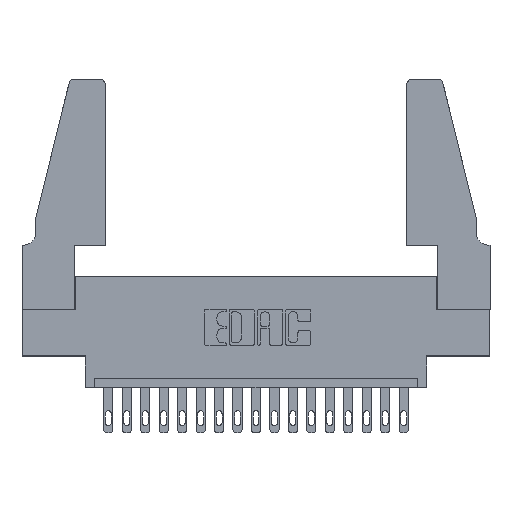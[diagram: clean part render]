
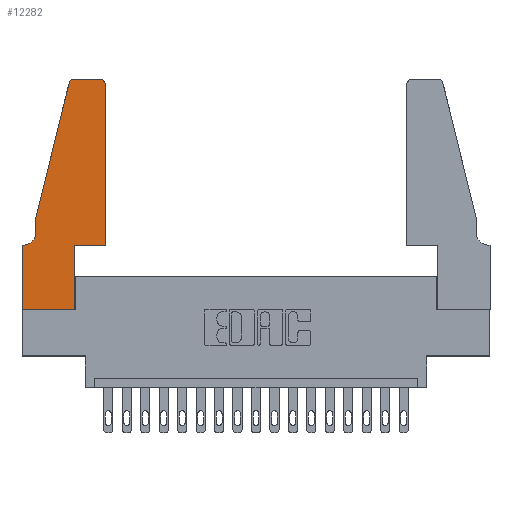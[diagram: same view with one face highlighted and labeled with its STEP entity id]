
A CAD part, top view. The second image highlights one B-rep face of the part: STEP entity #12282.
In plain terms, the highlighted planar face has unit normal (0, 0, 1).
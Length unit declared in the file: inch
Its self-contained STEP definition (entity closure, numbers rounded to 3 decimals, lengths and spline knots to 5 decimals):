
#371 = VECTOR ( 'NONE', #3608, 39.37008 ) ;
#410 = VERTEX_POINT ( 'NONE', #6914 ) ;
#624 = ORIENTED_EDGE ( 'NONE', *, *, #14106, .T. ) ;
#739 = CARTESIAN_POINT ( 'NONE',  ( 0.2865, 0.35, 0.37 ) ) ;
#763 = VERTEX_POINT ( 'NONE', #1610 ) ;
#771 = CARTESIAN_POINT ( 'NONE',  ( 0.4505, 0.35, 0.37 ) ) ;
#846 = LINE ( 'NONE', #1832, #3275 ) ;
#1291 = CARTESIAN_POINT ( 'NONE',  ( 0.0755, 0.5, 0.37 ) ) ;
#1357 = CARTESIAN_POINT ( 'NONE',  ( 0., 0., 0.37 ) ) ;
#1410 = CARTESIAN_POINT ( 'NONE',  ( 0.2865, 0.35, 0.37 ) ) ;
#1493 = CARTESIAN_POINT ( 'NONE',  ( 0.4505, 0.35, 0.37 ) ) ;
#1610 = CARTESIAN_POINT ( 'NONE',  ( 0.25487, 1.22718, 0.37 ) ) ;
#1832 = CARTESIAN_POINT ( 'NONE',  ( 0.2605, 1.25, 0.37 ) ) ;
#1954 = EDGE_CURVE ( 'NONE', #10099, #12650, #4703, .T. ) ;
#2339 = DIRECTION ( 'NONE',  ( 1., 0., 0. ) ) ;
#2361 = VECTOR ( 'NONE', #6829, 39.37008 ) ;
#2858 = ORIENTED_EDGE ( 'NONE', *, *, #18289, .T. ) ;
#3275 = VECTOR ( 'NONE', #7366, 39.37008 ) ;
#3564 = ORIENTED_EDGE ( 'NONE', *, *, #7827, .T. ) ;
#3608 = DIRECTION ( 'NONE',  ( 0., 1., 0. ) ) ;
#3781 = CARTESIAN_POINT ( 'NONE',  ( 0., 0., 0.37 ) ) ;
#3797 = AXIS2_PLACEMENT_3D ( 'NONE', #14997, #4817, #7934 ) ;
#4042 = LINE ( 'NONE', #10517, #10256 ) ;
#4330 = EDGE_CURVE ( 'NONE', #6242, #4493, #17198, .T. ) ;
#4493 = VERTEX_POINT ( 'NONE', #7048 ) ;
#4703 = CIRCLE ( 'NONE', #17591, 0.07 ) ;
#4817 = DIRECTION ( 'NONE',  ( 0., 0., 1. ) ) ;
#4842 = DIRECTION ( 'NONE',  ( 1., 0., 0. ) ) ;
#5022 = VECTOR ( 'NONE', #16848, 39.37008 ) ;
#5751 = LINE ( 'NONE', #18090, #9321 ) ;
#6242 = VERTEX_POINT ( 'NONE', #771 ) ;
#6408 = DIRECTION ( 'NONE',  ( 0., 0., 1. ) ) ;
#6492 = PLANE ( 'NONE',  #8115 ) ;
#6562 = VECTOR ( 'NONE', #10854, 39.37008 ) ;
#6829 = DIRECTION ( 'NONE',  ( -0.239, -0.971, 0. ) ) ;
#6858 = EDGE_CURVE ( 'NONE', #12650, #9502, #4042, .T. ) ;
#6914 = CARTESIAN_POINT ( 'NONE',  ( 0.284, 1.25, 0.37 ) ) ;
#7048 = CARTESIAN_POINT ( 'NONE',  ( 0.4505, 1.22, 0.37 ) ) ;
#7186 = CIRCLE ( 'NONE', #13896, 0.03 ) ;
#7366 = DIRECTION ( 'NONE',  ( -1., 0., 0. ) ) ;
#7744 = VERTEX_POINT ( 'NONE', #13415 ) ;
#7827 = EDGE_CURVE ( 'NONE', #8183, #6242, #5751, .T. ) ;
#7934 = DIRECTION ( 'NONE',  ( 1., 0., 0. ) ) ;
#8115 = AXIS2_PLACEMENT_3D ( 'NONE', #18087, #12432, #10954 ) ;
#8183 = VERTEX_POINT ( 'NONE', #1410 ) ;
#8214 = EDGE_CURVE ( 'NONE', #7744, #410, #846, .T. ) ;
#8449 = FACE_OUTER_BOUND ( 'NONE', #15818, .T. ) ;
#8538 = ORIENTED_EDGE ( 'NONE', *, *, #4330, .T. ) ;
#8615 = CARTESIAN_POINT ( 'NONE',  ( 0.0755, 0.42, 0.37 ) ) ;
#8864 = DIRECTION ( 'NONE',  ( 0., 1., 0. ) ) ;
#8883 = ORIENTED_EDGE ( 'NONE', *, *, #12436, .T. ) ;
#9064 = ORIENTED_EDGE ( 'NONE', *, *, #9768, .T. ) ;
#9321 = VECTOR ( 'NONE', #2339, 39.37008 ) ;
#9341 = VERTEX_POINT ( 'NONE', #17057 ) ;
#9502 = VERTEX_POINT ( 'NONE', #14697 ) ;
#9745 = EDGE_CURVE ( 'NONE', #410, #763, #9914, .T. ) ;
#9768 = EDGE_CURVE ( 'NONE', #763, #9341, #13198, .T. ) ;
#9914 = CIRCLE ( 'NONE', #3797, 0.03 ) ;
#9916 = DIRECTION ( 'NONE',  ( 0., -1., 0. ) ) ;
#10099 = VERTEX_POINT ( 'NONE', #8615 ) ;
#10124 = ORIENTED_EDGE ( 'NONE', *, *, #16951, .T. ) ;
#10141 = LINE ( 'NONE', #1357, #5022 ) ;
#10256 = VECTOR ( 'NONE', #11181, 39.37008 ) ;
#10488 = DIRECTION ( 'NONE',  ( 0., 0., -1. ) ) ;
#10517 = CARTESIAN_POINT ( 'NONE',  ( 0.0755, 0.35, 0.37 ) ) ;
#10627 = VERTEX_POINT ( 'NONE', #14741 ) ;
#10675 = EDGE_CURVE ( 'NONE', #4493, #7744, #7186, .T. ) ;
#10676 = ORIENTED_EDGE ( 'NONE', *, *, #10675, .T. ) ;
#10772 = VECTOR ( 'NONE', #8864, 39.37008 ) ;
#10849 = VECTOR ( 'NONE', #9916, 39.37008 ) ;
#10854 = DIRECTION ( 'NONE',  ( 1., 0., 0. ) ) ;
#10954 = DIRECTION ( 'NONE',  ( 1., 0., 0. ) ) ;
#11181 = DIRECTION ( 'NONE',  ( -1., 0., 0. ) ) ;
#11604 = DIRECTION ( 'NONE',  ( -1., 0., 0. ) ) ;
#12282 = ADVANCED_FACE ( 'NONE', ( #8449 ), #6492, .T. ) ;
#12309 = LINE ( 'NONE', #3781, #6562 ) ;
#12432 = DIRECTION ( 'NONE',  ( 0., 0., 1. ) ) ;
#12436 = EDGE_CURVE ( 'NONE', #9341, #10099, #16144, .T. ) ;
#12471 = ORIENTED_EDGE ( 'NONE', *, *, #1954, .T. ) ;
#12650 = VERTEX_POINT ( 'NONE', #14615 ) ;
#13198 = LINE ( 'NONE', #1291, #2361 ) ;
#13329 = VERTEX_POINT ( 'NONE', #16591 ) ;
#13415 = CARTESIAN_POINT ( 'NONE',  ( 0.4205, 1.25, 0.37 ) ) ;
#13453 = CARTESIAN_POINT ( 'NONE',  ( 0.4205, 1.22, 0.37 ) ) ;
#13896 = AXIS2_PLACEMENT_3D ( 'NONE', #13453, #6408, #4842 ) ;
#14106 = EDGE_CURVE ( 'NONE', #9502, #10627, #10141, .T. ) ;
#14281 = ORIENTED_EDGE ( 'NONE', *, *, #8214, .T. ) ;
#14551 = CARTESIAN_POINT ( 'NONE',  ( 0.0055, 0.42, 0.37 ) ) ;
#14615 = CARTESIAN_POINT ( 'NONE',  ( 0.0055, 0.35, 0.37 ) ) ;
#14697 = CARTESIAN_POINT ( 'NONE',  ( 0., 0.35, 0.37 ) ) ;
#14741 = CARTESIAN_POINT ( 'NONE',  ( 0., 0., 0.37 ) ) ;
#14997 = CARTESIAN_POINT ( 'NONE',  ( 0.284, 1.22, 0.37 ) ) ;
#15818 = EDGE_LOOP ( 'NONE', ( #14281, #16365, #9064, #8883, #12471, #16768, #624, #2858, #10124, #3564, #8538, #10676 ) ) ;
#15887 = LINE ( 'NONE', #739, #371 ) ;
#16144 = LINE ( 'NONE', #18342, #10849 ) ;
#16365 = ORIENTED_EDGE ( 'NONE', *, *, #9745, .T. ) ;
#16591 = CARTESIAN_POINT ( 'NONE',  ( 0.2865, 0., 0.37 ) ) ;
#16768 = ORIENTED_EDGE ( 'NONE', *, *, #6858, .T. ) ;
#16848 = DIRECTION ( 'NONE',  ( 0., -1., 0. ) ) ;
#16951 = EDGE_CURVE ( 'NONE', #13329, #8183, #15887, .T. ) ;
#17057 = CARTESIAN_POINT ( 'NONE',  ( 0.0755, 0.5, 0.37 ) ) ;
#17198 = LINE ( 'NONE', #1493, #10772 ) ;
#17591 = AXIS2_PLACEMENT_3D ( 'NONE', #14551, #10488, #11604 ) ;
#18087 = CARTESIAN_POINT ( 'NONE',  ( 0., 0.35, 0.37 ) ) ;
#18090 = CARTESIAN_POINT ( 'NONE',  ( 0.4505, 0.35, 0.37 ) ) ;
#18289 = EDGE_CURVE ( 'NONE', #10627, #13329, #12309, .T. ) ;
#18342 = CARTESIAN_POINT ( 'NONE',  ( 0.0755, 0.5, 0.37 ) ) ;
